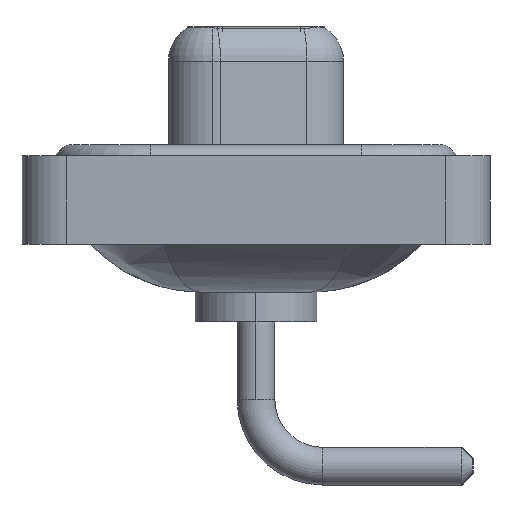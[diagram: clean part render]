
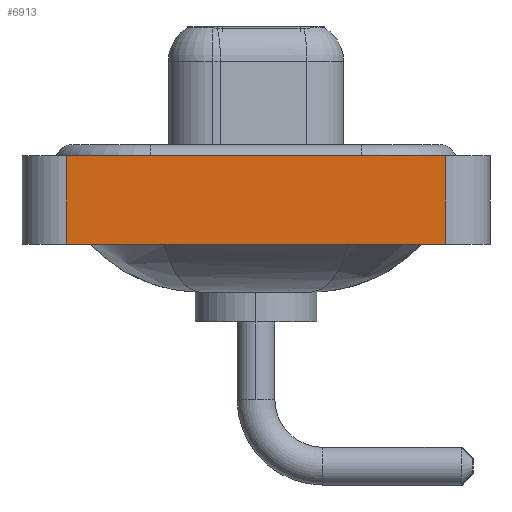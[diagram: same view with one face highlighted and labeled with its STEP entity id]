
A CAD part, left-side view. The second image highlights one B-rep face of the part: STEP entity #6913.
In plain terms, the highlighted planar face has unit normal (-1, 0, 0).
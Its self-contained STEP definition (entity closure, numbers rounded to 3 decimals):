
#218 = CARTESIAN_POINT ( 'NONE',  ( -7.3, 8.55, -3.6 ) ) ;
#723 = DIRECTION ( 'NONE',  ( -1., 0., 0. ) ) ;
#760 = VERTEX_POINT ( 'NONE', #6071 ) ;
#967 = VECTOR ( 'NONE', #13405, 1000. ) ;
#1222 = EDGE_CURVE ( 'NONE', #760, #6617, #4641, .T. ) ;
#1886 = ORIENTED_EDGE ( 'NONE', *, *, #11851, .F. ) ;
#3222 = LINE ( 'NONE', #12719, #16742 ) ;
#4152 = EDGE_CURVE ( 'NONE', #13584, #760, #8860, .T. ) ;
#4641 = LINE ( 'NONE', #9934, #9341 ) ;
#4760 = DIRECTION ( 'NONE',  ( 0., 0., 1. ) ) ;
#6071 = CARTESIAN_POINT ( 'NONE',  ( -7.3, -8.55, -3.6 ) ) ;
#6180 = VECTOR ( 'NONE', #6272, 1000. ) ;
#6272 = DIRECTION ( 'NONE',  ( 0., -1., 0. ) ) ;
#6295 = CARTESIAN_POINT ( 'NONE',  ( -7.3, -8.55, 0.4 ) ) ;
#6469 = LINE ( 'NONE', #11838, #967 ) ;
#6617 = VERTEX_POINT ( 'NONE', #6295 ) ;
#6877 = ORIENTED_EDGE ( 'NONE', *, *, #16743, .F. ) ;
#6913 = ADVANCED_FACE ( 'NONE', ( #15560 ), #9084, .T. ) ;
#7408 = CARTESIAN_POINT ( 'NONE',  ( -7.3, -8.55, -3.6 ) ) ;
#7429 = EDGE_LOOP ( 'NONE', ( #12730, #6877, #1886, #8692 ) ) ;
#8692 = ORIENTED_EDGE ( 'NONE', *, *, #4152, .T. ) ;
#8860 = LINE ( 'NONE', #11570, #6180 ) ;
#9084 = PLANE ( 'NONE',  #9900 ) ;
#9341 = VECTOR ( 'NONE', #14136, 1000. ) ;
#9900 = AXIS2_PLACEMENT_3D ( 'NONE', #7408, #723, #4760 ) ;
#9934 = CARTESIAN_POINT ( 'NONE',  ( -7.3, -8.55, -3.6 ) ) ;
#10001 = DIRECTION ( 'NONE',  ( 0., -1., 0. ) ) ;
#11570 = CARTESIAN_POINT ( 'NONE',  ( -7.3, -8.55, -3.6 ) ) ;
#11838 = CARTESIAN_POINT ( 'NONE',  ( -7.3, 8.55, -3.6 ) ) ;
#11851 = EDGE_CURVE ( 'NONE', #13584, #16823, #6469, .T. ) ;
#11914 = CARTESIAN_POINT ( 'NONE',  ( -7.3, 8.55, 0.4 ) ) ;
#12719 = CARTESIAN_POINT ( 'NONE',  ( -7.3, -8.55, 0.4 ) ) ;
#12730 = ORIENTED_EDGE ( 'NONE', *, *, #1222, .T. ) ;
#13405 = DIRECTION ( 'NONE',  ( 0., 0., 1. ) ) ;
#13584 = VERTEX_POINT ( 'NONE', #218 ) ;
#14136 = DIRECTION ( 'NONE',  ( 0., 0., 1. ) ) ;
#15560 = FACE_OUTER_BOUND ( 'NONE', #7429, .T. ) ;
#16742 = VECTOR ( 'NONE', #10001, 1000. ) ;
#16743 = EDGE_CURVE ( 'NONE', #16823, #6617, #3222, .T. ) ;
#16823 = VERTEX_POINT ( 'NONE', #11914 ) ;
